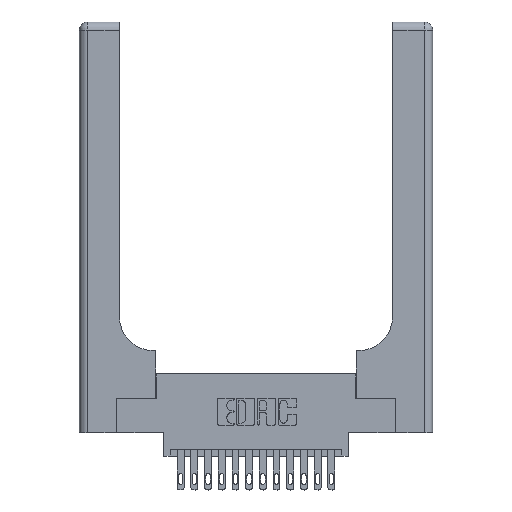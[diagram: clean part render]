
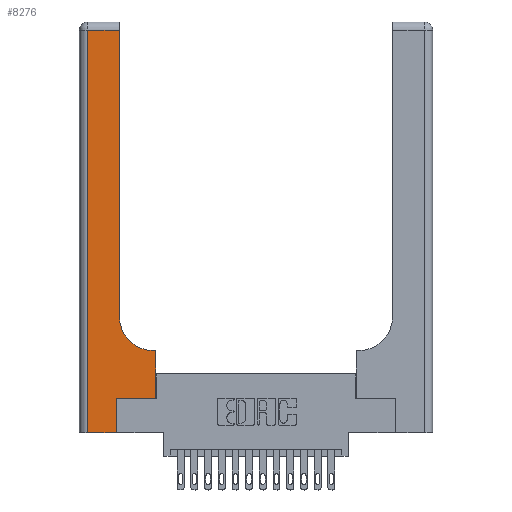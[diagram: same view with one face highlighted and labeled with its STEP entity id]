
A CAD part, top view. The second image highlights one B-rep face of the part: STEP entity #8276.
In plain terms, the highlighted planar face has unit normal (0, 0, 1).
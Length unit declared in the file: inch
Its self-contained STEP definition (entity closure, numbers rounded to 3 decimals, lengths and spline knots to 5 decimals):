
#244 = EDGE_CURVE ( 'NONE', #2551, #5752, #12874, .T. ) ;
#1233 = AXIS2_PLACEMENT_3D ( 'NONE', #4649, #17649, #14749 ) ;
#1272 = LINE ( 'NONE', #4161, #13865 ) ;
#1827 = DIRECTION ( 'NONE',  ( -1., 0., 0. ) ) ;
#1951 = LINE ( 'NONE', #3129, #9166 ) ;
#2064 = LINE ( 'NONE', #14152, #15379 ) ;
#2251 = DIRECTION ( 'NONE',  ( 0., 0., -1. ) ) ;
#2412 = VERTEX_POINT ( 'NONE', #6989 ) ;
#2551 = VERTEX_POINT ( 'NONE', #18248 ) ;
#2606 = DIRECTION ( 'NONE',  ( 0., 1., 0. ) ) ;
#2709 = DIRECTION ( 'NONE',  ( 0., -1., 0. ) ) ;
#2719 = DIRECTION ( 'NONE',  ( -1., 0., 0. ) ) ;
#2836 = VERTEX_POINT ( 'NONE', #17949 ) ;
#3117 = ORIENTED_EDGE ( 'NONE', *, *, #13443, .T. ) ;
#3129 = CARTESIAN_POINT ( 'NONE',  ( 0.2915, 0.6, 0.37 ) ) ;
#3387 = DIRECTION ( 'NONE',  ( 0., 1., 0. ) ) ;
#4077 = ORIENTED_EDGE ( 'NONE', *, *, #8371, .T. ) ;
#4161 = CARTESIAN_POINT ( 'NONE',  ( 0.06, 3., 0.37 ) ) ;
#4481 = EDGE_CURVE ( 'NONE', #18576, #2412, #1272, .T. ) ;
#4649 = CARTESIAN_POINT ( 'NONE',  ( 0.5415, 0.85, 0.37 ) ) ;
#4927 = EDGE_LOOP ( 'NONE', ( #3117, #8416, #17384, #10838, #4077, #12418, #17814, #6763, #8354 ) ) ;
#5148 = CARTESIAN_POINT ( 'NONE',  ( 0.06, 2.94, 0.37 ) ) ;
#5621 = CARTESIAN_POINT ( 'NONE',  ( 0.5585, 0.25, 0.37 ) ) ;
#5752 = VERTEX_POINT ( 'NONE', #7772 ) ;
#5782 = VECTOR ( 'NONE', #13162, 39.37008 ) ;
#6196 = CARTESIAN_POINT ( 'NONE',  ( 0., 0., 0.37 ) ) ;
#6726 = CARTESIAN_POINT ( 'NONE',  ( 0.269, 0.25, 0.37 ) ) ;
#6763 = ORIENTED_EDGE ( 'NONE', *, *, #15726, .T. ) ;
#6989 = CARTESIAN_POINT ( 'NONE',  ( 0.06, 0., 0.37 ) ) ;
#6991 = DIRECTION ( 'NONE',  ( 0., 1., 0. ) ) ;
#7727 = DIRECTION ( 'NONE',  ( 1., 0., 0. ) ) ;
#7772 = CARTESIAN_POINT ( 'NONE',  ( 0.5585, 0.6, 0.37 ) ) ;
#7907 = LINE ( 'NONE', #10506, #10604 ) ;
#7929 = CARTESIAN_POINT ( 'NONE',  ( 0., 3., 0.37 ) ) ;
#8101 = VECTOR ( 'NONE', #7727, 39.37008 ) ;
#8276 = ADVANCED_FACE ( 'NONE', ( #8395 ), #16596, .F. ) ;
#8354 = ORIENTED_EDGE ( 'NONE', *, *, #18297, .T. ) ;
#8371 = EDGE_CURVE ( 'NONE', #18231, #18581, #2064, .T. ) ;
#8395 = FACE_OUTER_BOUND ( 'NONE', #4927, .T. ) ;
#8411 = CARTESIAN_POINT ( 'NONE',  ( 0.5415, 0.6, 0.37 ) ) ;
#8416 = ORIENTED_EDGE ( 'NONE', *, *, #16761, .T. ) ;
#9166 = VECTOR ( 'NONE', #1827, 39.37008 ) ;
#9529 = VERTEX_POINT ( 'NONE', #8411 ) ;
#9909 = LINE ( 'NONE', #6196, #8101 ) ;
#10149 = CARTESIAN_POINT ( 'NONE',  ( 0.269, 0., 0.37 ) ) ;
#10294 = LINE ( 'NONE', #16046, #5782 ) ;
#10506 = CARTESIAN_POINT ( 'NONE',  ( 0.2915, 3., 0.37 ) ) ;
#10604 = VECTOR ( 'NONE', #3387, 39.37008 ) ;
#10838 = ORIENTED_EDGE ( 'NONE', *, *, #14163, .T. ) ;
#11920 = CARTESIAN_POINT ( 'NONE',  ( 0.2915, 2.94, 0.37 ) ) ;
#12177 = EDGE_CURVE ( 'NONE', #18581, #2551, #10294, .T. ) ;
#12418 = ORIENTED_EDGE ( 'NONE', *, *, #12177, .T. ) ;
#12874 = LINE ( 'NONE', #5621, #16990 ) ;
#13162 = DIRECTION ( 'NONE',  ( 1., 0., 0. ) ) ;
#13286 = AXIS2_PLACEMENT_3D ( 'NONE', #7929, #2251, #13693 ) ;
#13422 = VERTEX_POINT ( 'NONE', #11920 ) ;
#13443 = EDGE_CURVE ( 'NONE', #2836, #13422, #7907, .T. ) ;
#13553 = CIRCLE ( 'NONE', #1233, 0.25 ) ;
#13693 = DIRECTION ( 'NONE',  ( -1., 0., 0. ) ) ;
#13865 = VECTOR ( 'NONE', #2709, 39.37008 ) ;
#14066 = LINE ( 'NONE', #15468, #18204 ) ;
#14152 = CARTESIAN_POINT ( 'NONE',  ( 0.269, 0., 0.37 ) ) ;
#14163 = EDGE_CURVE ( 'NONE', #2412, #18231, #9909, .T. ) ;
#14749 = DIRECTION ( 'NONE',  ( 1., 0., 0. ) ) ;
#15379 = VECTOR ( 'NONE', #6991, 39.37008 ) ;
#15468 = CARTESIAN_POINT ( 'NONE',  ( 0., 2.94, 0.37 ) ) ;
#15726 = EDGE_CURVE ( 'NONE', #5752, #9529, #1951, .T. ) ;
#16046 = CARTESIAN_POINT ( 'NONE',  ( 0.269, 0.25, 0.37 ) ) ;
#16596 = PLANE ( 'NONE',  #13286 ) ;
#16761 = EDGE_CURVE ( 'NONE', #13422, #18576, #14066, .T. ) ;
#16990 = VECTOR ( 'NONE', #2606, 39.37008 ) ;
#17384 = ORIENTED_EDGE ( 'NONE', *, *, #4481, .T. ) ;
#17649 = DIRECTION ( 'NONE',  ( 0., 0., -1. ) ) ;
#17814 = ORIENTED_EDGE ( 'NONE', *, *, #244, .T. ) ;
#17949 = CARTESIAN_POINT ( 'NONE',  ( 0.2915, 0.85, 0.37 ) ) ;
#18204 = VECTOR ( 'NONE', #2719, 39.37008 ) ;
#18231 = VERTEX_POINT ( 'NONE', #10149 ) ;
#18248 = CARTESIAN_POINT ( 'NONE',  ( 0.5585, 0.25, 0.37 ) ) ;
#18297 = EDGE_CURVE ( 'NONE', #9529, #2836, #13553, .T. ) ;
#18576 = VERTEX_POINT ( 'NONE', #5148 ) ;
#18581 = VERTEX_POINT ( 'NONE', #6726 ) ;
